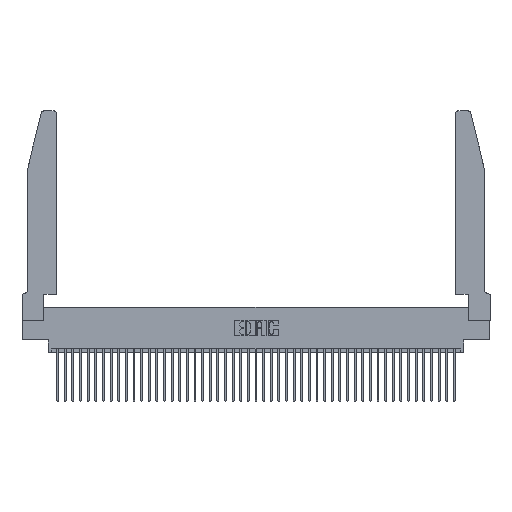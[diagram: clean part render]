
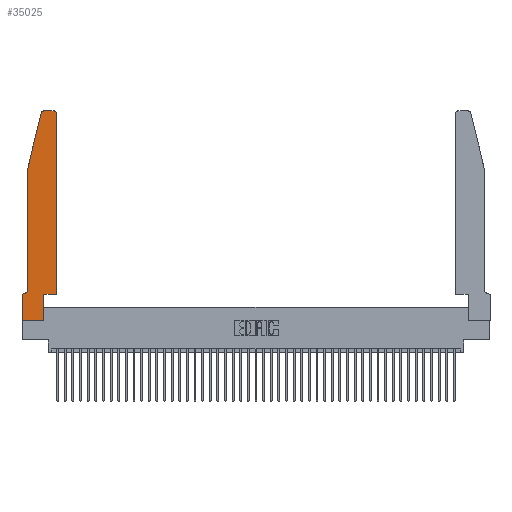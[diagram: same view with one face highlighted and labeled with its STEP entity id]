
A CAD part, top view. The second image highlights one B-rep face of the part: STEP entity #35025.
In plain terms, the highlighted planar face has unit normal (0, 0, 1).
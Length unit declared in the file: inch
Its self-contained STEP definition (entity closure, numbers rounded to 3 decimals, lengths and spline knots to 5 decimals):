
#33 = VERTEX_POINT ( 'NONE', #1833 ) ;
#599 = CARTESIAN_POINT ( 'NONE',  ( 0.2865, 0., 0.37 ) ) ;
#689 = VERTEX_POINT ( 'NONE', #599 ) ;
#1102 = EDGE_CURVE ( 'NONE', #37767, #33, #20609, .T. ) ;
#1157 = VERTEX_POINT ( 'NONE', #23074 ) ;
#1322 = CARTESIAN_POINT ( 'NONE',  ( 0., 0.35, 0.37 ) ) ;
#1622 = DIRECTION ( 'NONE',  ( 0., 0., 1. ) ) ;
#1833 = CARTESIAN_POINT ( 'NONE',  ( 0.0755, 0.42, 0.37 ) ) ;
#2538 = VECTOR ( 'NONE', #41443, 39.37008 ) ;
#2615 = CARTESIAN_POINT ( 'NONE',  ( 0.4505, 0.35, 0.37 ) ) ;
#2912 = ORIENTED_EDGE ( 'NONE', *, *, #9473, .T. ) ;
#3177 = EDGE_CURVE ( 'NONE', #29890, #30980, #5279, .T. ) ;
#3855 = CARTESIAN_POINT ( 'NONE',  ( 0.2865, 0.35, 0.37 ) ) ;
#4632 = CARTESIAN_POINT ( 'NONE',  ( 0.284, 2.75, 0.37 ) ) ;
#4789 = DIRECTION ( 'NONE',  ( 1., 0., 0. ) ) ;
#5279 = LINE ( 'NONE', #27158, #2538 ) ;
#5460 = DIRECTION ( 'NONE',  ( 0., -1., 0. ) ) ;
#5912 = AXIS2_PLACEMENT_3D ( 'NONE', #42984, #1622, #4789 ) ;
#6398 = VERTEX_POINT ( 'NONE', #31314 ) ;
#6605 = VERTEX_POINT ( 'NONE', #36920 ) ;
#6859 = EDGE_CURVE ( 'NONE', #1157, #689, #12631, .T. ) ;
#8080 = VECTOR ( 'NONE', #5460, 39.37008 ) ;
#9473 = EDGE_CURVE ( 'NONE', #6605, #37767, #37360, .T. ) ;
#9512 = VERTEX_POINT ( 'NONE', #11527 ) ;
#9645 = CARTESIAN_POINT ( 'NONE',  ( 0.0755, 2., 0.37 ) ) ;
#11449 = FACE_OUTER_BOUND ( 'NONE', #35252, .T. ) ;
#11527 = CARTESIAN_POINT ( 'NONE',  ( 0.4505, 2.72, 0.37 ) ) ;
#11572 = CARTESIAN_POINT ( 'NONE',  ( 0., 0., 0.37 ) ) ;
#12188 = VECTOR ( 'NONE', #25902, 39.37008 ) ;
#12582 = CARTESIAN_POINT ( 'NONE',  ( 0.284, 2.72, 0.37 ) ) ;
#12631 = LINE ( 'NONE', #11572, #23402 ) ;
#13040 = ORIENTED_EDGE ( 'NONE', *, *, #30479, .T. ) ;
#13724 = AXIS2_PLACEMENT_3D ( 'NONE', #12582, #37757, #44855 ) ;
#13978 = CARTESIAN_POINT ( 'NONE',  ( 0.4205, 2.75, 0.37 ) ) ;
#14065 = CARTESIAN_POINT ( 'NONE',  ( 0.4505, 0.35, 0.37 ) ) ;
#14155 = CARTESIAN_POINT ( 'NONE',  ( 0., 0., 0.37 ) ) ;
#14496 = VERTEX_POINT ( 'NONE', #1322 ) ;
#14827 = CARTESIAN_POINT ( 'NONE',  ( 0.0055, 0.42, 0.37 ) ) ;
#15017 = DIRECTION ( 'NONE',  ( 1., 0., 0. ) ) ;
#16194 = ORIENTED_EDGE ( 'NONE', *, *, #39566, .T. ) ;
#16276 = ORIENTED_EDGE ( 'NONE', *, *, #1102, .T. ) ;
#17337 = EDGE_CURVE ( 'NONE', #30980, #6605, #26652, .T. ) ;
#17504 = DIRECTION ( 'NONE',  ( 1., 0., 0. ) ) ;
#18643 = VERTEX_POINT ( 'NONE', #2615 ) ;
#19433 = CARTESIAN_POINT ( 'NONE',  ( 0.0755, 2., 0.37 ) ) ;
#19798 = ORIENTED_EDGE ( 'NONE', *, *, #32798, .T. ) ;
#20331 = VECTOR ( 'NONE', #28180, 39.37008 ) ;
#20337 = LINE ( 'NONE', #41914, #26899 ) ;
#20609 = LINE ( 'NONE', #19433, #8080 ) ;
#21532 = CIRCLE ( 'NONE', #5912, 0.03 ) ;
#22588 = VERTEX_POINT ( 'NONE', #39614 ) ;
#22982 = LINE ( 'NONE', #14065, #27307 ) ;
#23074 = CARTESIAN_POINT ( 'NONE',  ( 0., 0., 0.37 ) ) ;
#23402 = VECTOR ( 'NONE', #31894, 39.37008 ) ;
#23711 = ORIENTED_EDGE ( 'NONE', *, *, #31432, .T. ) ;
#24591 = ORIENTED_EDGE ( 'NONE', *, *, #17337, .T. ) ;
#25902 = DIRECTION ( 'NONE',  ( -1., 0., 0. ) ) ;
#26514 = CARTESIAN_POINT ( 'NONE',  ( 0.0755, 0.35, 0.37 ) ) ;
#26652 = CIRCLE ( 'NONE', #13724, 0.03 ) ;
#26899 = VECTOR ( 'NONE', #15017, 39.37008 ) ;
#27158 = CARTESIAN_POINT ( 'NONE',  ( 0.2605, 2.75, 0.37 ) ) ;
#27307 = VECTOR ( 'NONE', #27705, 39.37008 ) ;
#27665 = PLANE ( 'NONE',  #33032 ) ;
#27705 = DIRECTION ( 'NONE',  ( 0., 1., 0. ) ) ;
#28180 = DIRECTION ( 'NONE',  ( 0., 1., 0. ) ) ;
#29174 = AXIS2_PLACEMENT_3D ( 'NONE', #14827, #39085, #32376 ) ;
#29890 = VERTEX_POINT ( 'NONE', #13978 ) ;
#29988 = LINE ( 'NONE', #14155, #35347 ) ;
#30479 = EDGE_CURVE ( 'NONE', #18643, #9512, #22982, .T. ) ;
#30897 = EDGE_CURVE ( 'NONE', #9512, #29890, #21532, .T. ) ;
#30980 = VERTEX_POINT ( 'NONE', #4632 ) ;
#30986 = DIRECTION ( 'NONE',  ( 0., -1., 0. ) ) ;
#31314 = CARTESIAN_POINT ( 'NONE',  ( 0.2865, 0.35, 0.37 ) ) ;
#31432 = EDGE_CURVE ( 'NONE', #33, #22588, #32916, .T. ) ;
#31894 = DIRECTION ( 'NONE',  ( 1., 0., 0. ) ) ;
#32376 = DIRECTION ( 'NONE',  ( -1., 0., 0. ) ) ;
#32611 = DIRECTION ( 'NONE',  ( -0.239, -0.971, 0. ) ) ;
#32798 = EDGE_CURVE ( 'NONE', #6398, #18643, #20337, .T. ) ;
#32916 = CIRCLE ( 'NONE', #29174, 0.07 ) ;
#33032 = AXIS2_PLACEMENT_3D ( 'NONE', #34778, #38306, #17504 ) ;
#33361 = ORIENTED_EDGE ( 'NONE', *, *, #30897, .T. ) ;
#33538 = VECTOR ( 'NONE', #32611, 39.37008 ) ;
#33883 = LINE ( 'NONE', #26514, #12188 ) ;
#34627 = ORIENTED_EDGE ( 'NONE', *, *, #39246, .T. ) ;
#34778 = CARTESIAN_POINT ( 'NONE',  ( 0., 0.35, 0.37 ) ) ;
#35025 = ADVANCED_FACE ( 'NONE', ( #11449 ), #27665, .T. ) ;
#35252 = EDGE_LOOP ( 'NONE', ( #37472, #24591, #2912, #16276, #23711, #16194, #40475, #41433, #34627, #19798, #13040, #33361 ) ) ;
#35347 = VECTOR ( 'NONE', #30986, 39.37008 ) ;
#36920 = CARTESIAN_POINT ( 'NONE',  ( 0.25487, 2.72718, 0.37 ) ) ;
#37360 = LINE ( 'NONE', #39166, #33538 ) ;
#37472 = ORIENTED_EDGE ( 'NONE', *, *, #3177, .T. ) ;
#37757 = DIRECTION ( 'NONE',  ( 0., 0., 1. ) ) ;
#37767 = VERTEX_POINT ( 'NONE', #9645 ) ;
#38306 = DIRECTION ( 'NONE',  ( 0., 0., 1. ) ) ;
#39085 = DIRECTION ( 'NONE',  ( 0., 0., -1. ) ) ;
#39166 = CARTESIAN_POINT ( 'NONE',  ( 0.0755, 2., 0.37 ) ) ;
#39246 = EDGE_CURVE ( 'NONE', #689, #6398, #43771, .T. ) ;
#39566 = EDGE_CURVE ( 'NONE', #22588, #14496, #33883, .T. ) ;
#39614 = CARTESIAN_POINT ( 'NONE',  ( 0.0055, 0.35, 0.37 ) ) ;
#40475 = ORIENTED_EDGE ( 'NONE', *, *, #40958, .T. ) ;
#40958 = EDGE_CURVE ( 'NONE', #14496, #1157, #29988, .T. ) ;
#41433 = ORIENTED_EDGE ( 'NONE', *, *, #6859, .T. ) ;
#41443 = DIRECTION ( 'NONE',  ( -1., 0., 0. ) ) ;
#41914 = CARTESIAN_POINT ( 'NONE',  ( 0.4505, 0.35, 0.37 ) ) ;
#42984 = CARTESIAN_POINT ( 'NONE',  ( 0.4205, 2.72, 0.37 ) ) ;
#43771 = LINE ( 'NONE', #3855, #20331 ) ;
#44855 = DIRECTION ( 'NONE',  ( 1., 0., 0. ) ) ;
